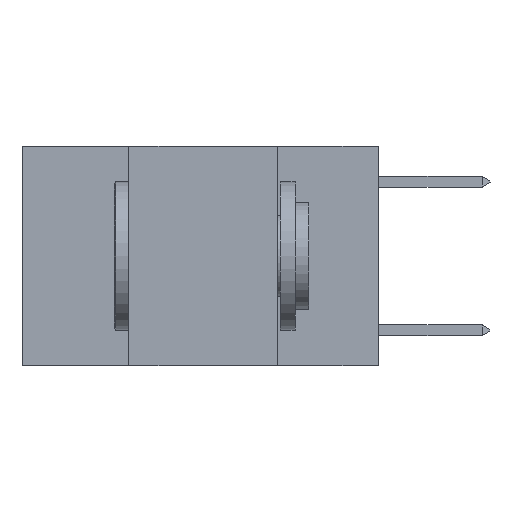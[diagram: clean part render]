
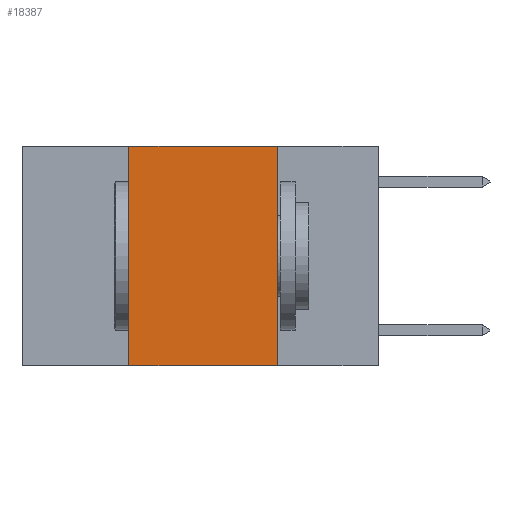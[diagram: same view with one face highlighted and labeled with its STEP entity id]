
A CAD part, left-side view. The second image highlights one B-rep face of the part: STEP entity #18387.
In plain terms, the highlighted planar face has unit normal (-1, 0, 0).
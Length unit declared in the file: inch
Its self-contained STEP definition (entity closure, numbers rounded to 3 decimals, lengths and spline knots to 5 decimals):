
#226 = DIRECTION ( 'NONE',  ( 0., 0., -1. ) ) ;
#1163 = LINE ( 'NONE', #18532, #4910 ) ;
#1292 = FACE_OUTER_BOUND ( 'NONE', #10658, .T. ) ;
#2168 = ORIENTED_EDGE ( 'NONE', *, *, #5051, .F. ) ;
#2799 = CARTESIAN_POINT ( 'NONE',  ( 0., 0.17, 0. ) ) ;
#2875 = DIRECTION ( 'NONE',  ( 0., -1., 0. ) ) ;
#3005 = CARTESIAN_POINT ( 'NONE',  ( 0., 0.42, -0.37 ) ) ;
#3074 = CARTESIAN_POINT ( 'NONE',  ( 0., 0.42, 0. ) ) ;
#3474 = ORIENTED_EDGE ( 'NONE', *, *, #22027, .T. ) ;
#4910 = VECTOR ( 'NONE', #2875, 39.37008 ) ;
#5009 = DIRECTION ( 'NONE',  ( 0., -1., 0. ) ) ;
#5051 = EDGE_CURVE ( 'NONE', #12141, #18328, #19052, .T. ) ;
#6498 = DIRECTION ( 'NONE',  ( 0., 0., -1. ) ) ;
#6699 = CARTESIAN_POINT ( 'NONE',  ( 0., 0.6, -0.37 ) ) ;
#7479 = AXIS2_PLACEMENT_3D ( 'NONE', #20128, #15224, #6498 ) ;
#8239 = PLANE ( 'NONE',  #7479 ) ;
#10474 = CARTESIAN_POINT ( 'NONE',  ( 0., 0.17, -0.37 ) ) ;
#10658 = EDGE_LOOP ( 'NONE', ( #16891, #17006, #2168, #3474 ) ) ;
#11027 = VECTOR ( 'NONE', #5009, 39.37008 ) ;
#11897 = CARTESIAN_POINT ( 'NONE',  ( 0., 0.42, 0. ) ) ;
#12035 = VECTOR ( 'NONE', #13480, 39.37008 ) ;
#12141 = VERTEX_POINT ( 'NONE', #3005 ) ;
#12938 = VECTOR ( 'NONE', #226, 39.37008 ) ;
#13480 = DIRECTION ( 'NONE',  ( 0., 0., 1. ) ) ;
#14279 = LINE ( 'NONE', #17805, #12938 ) ;
#15224 = DIRECTION ( 'NONE',  ( 1., 0., 0. ) ) ;
#16891 = ORIENTED_EDGE ( 'NONE', *, *, #17742, .F. ) ;
#17006 = ORIENTED_EDGE ( 'NONE', *, *, #18275, .F. ) ;
#17742 = EDGE_CURVE ( 'NONE', #19616, #20656, #14279, .T. ) ;
#17805 = CARTESIAN_POINT ( 'NONE',  ( 0., 0.17, 0. ) ) ;
#18275 = EDGE_CURVE ( 'NONE', #18328, #19616, #1163, .T. ) ;
#18328 = VERTEX_POINT ( 'NONE', #11897 ) ;
#18387 = ADVANCED_FACE ( 'NONE', ( #1292 ), #8239, .F. ) ;
#18532 = CARTESIAN_POINT ( 'NONE',  ( 0., 0.6, 0. ) ) ;
#19052 = LINE ( 'NONE', #3074, #12035 ) ;
#19616 = VERTEX_POINT ( 'NONE', #2799 ) ;
#20128 = CARTESIAN_POINT ( 'NONE',  ( 0., 0.6, 0. ) ) ;
#20656 = VERTEX_POINT ( 'NONE', #10474 ) ;
#20671 = LINE ( 'NONE', #6699, #11027 ) ;
#22027 = EDGE_CURVE ( 'NONE', #12141, #20656, #20671, .T. ) ;
